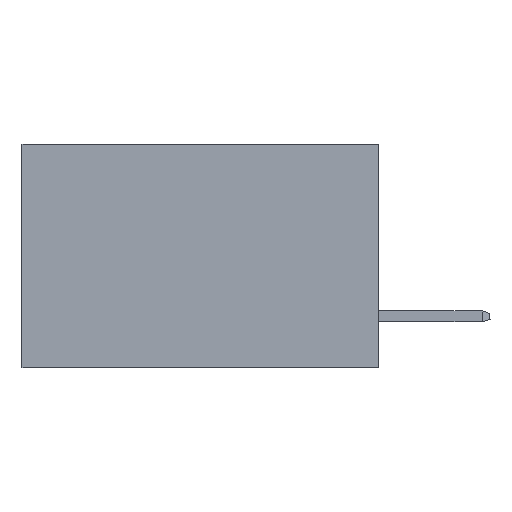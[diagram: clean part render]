
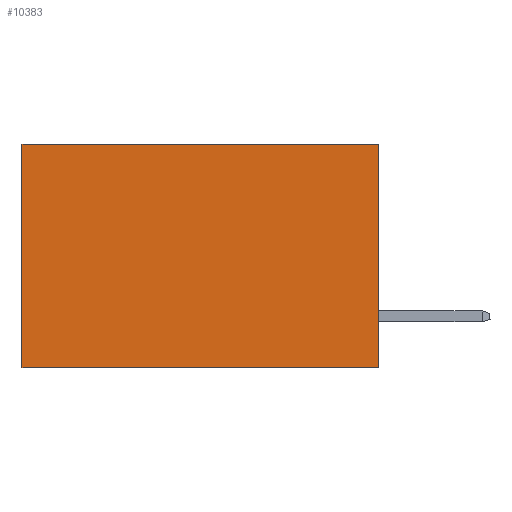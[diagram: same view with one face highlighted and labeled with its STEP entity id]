
A CAD part, left-side view. The second image highlights one B-rep face of the part: STEP entity #10383.
In plain terms, the highlighted planar face has unit normal (-1, 0, 0).
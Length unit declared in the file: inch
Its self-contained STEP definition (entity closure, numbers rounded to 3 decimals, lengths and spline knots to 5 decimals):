
#186 = LINE ( 'NONE', #8048, #23563 ) ;
#542 = DIRECTION ( 'NONE',  ( 0., 0., -1. ) ) ;
#1383 = DIRECTION ( 'NONE',  ( 1., 0., 0. ) ) ;
#2556 = AXIS2_PLACEMENT_3D ( 'NONE', #6354, #1383, #23823 ) ;
#4753 = CARTESIAN_POINT ( 'NONE',  ( 0.277, 0., 0. ) ) ;
#6354 = CARTESIAN_POINT ( 'NONE',  ( 0.277, 0., -0.37 ) ) ;
#8048 = CARTESIAN_POINT ( 'NONE',  ( 0.277, 0., -0.37 ) ) ;
#8263 = VERTEX_POINT ( 'NONE', #22224 ) ;
#8755 = PLANE ( 'NONE',  #2556 ) ;
#8800 = ORIENTED_EDGE ( 'NONE', *, *, #22665, .T. ) ;
#9054 = EDGE_CURVE ( 'NONE', #21464, #21645, #18186, .T. ) ;
#9182 = ORIENTED_EDGE ( 'NONE', *, *, #14695, .F. ) ;
#9859 = ORIENTED_EDGE ( 'NONE', *, *, #22012, .F. ) ;
#10264 = VERTEX_POINT ( 'NONE', #21380 ) ;
#10383 = ADVANCED_FACE ( 'NONE', ( #13274 ), #8755, .F. ) ;
#10411 = CARTESIAN_POINT ( 'NONE',  ( 0.277, 0.59, 0. ) ) ;
#13274 = FACE_OUTER_BOUND ( 'NONE', #14741, .T. ) ;
#13342 = VECTOR ( 'NONE', #13532, 39.37008 ) ;
#13532 = DIRECTION ( 'NONE',  ( 0., 0., -1. ) ) ;
#13721 = VECTOR ( 'NONE', #15578, 39.37008 ) ;
#13754 = CARTESIAN_POINT ( 'NONE',  ( 0.277, 0., -0.37 ) ) ;
#13959 = CARTESIAN_POINT ( 'NONE',  ( 0.277, 0.59, -0.37 ) ) ;
#14559 = VECTOR ( 'NONE', #19463, 39.37008 ) ;
#14695 = EDGE_CURVE ( 'NONE', #8263, #10264, #186, .T. ) ;
#14741 = EDGE_LOOP ( 'NONE', ( #23650, #9859, #9182, #8800 ) ) ;
#15114 = LINE ( 'NONE', #4753, #14559 ) ;
#15578 = DIRECTION ( 'NONE',  ( 0., 1., 0. ) ) ;
#16402 = CARTESIAN_POINT ( 'NONE',  ( 0.277, 0.59, -0.37 ) ) ;
#18186 = LINE ( 'NONE', #13959, #13342 ) ;
#19463 = DIRECTION ( 'NONE',  ( 0., 1., 0. ) ) ;
#21380 = CARTESIAN_POINT ( 'NONE',  ( 0.277, 0., -0.37 ) ) ;
#21464 = VERTEX_POINT ( 'NONE', #10411 ) ;
#21645 = VERTEX_POINT ( 'NONE', #16402 ) ;
#22012 = EDGE_CURVE ( 'NONE', #10264, #21645, #23341, .T. ) ;
#22224 = CARTESIAN_POINT ( 'NONE',  ( 0.277, 0., 0. ) ) ;
#22665 = EDGE_CURVE ( 'NONE', #8263, #21464, #15114, .T. ) ;
#23341 = LINE ( 'NONE', #13754, #13721 ) ;
#23563 = VECTOR ( 'NONE', #542, 39.37008 ) ;
#23650 = ORIENTED_EDGE ( 'NONE', *, *, #9054, .T. ) ;
#23823 = DIRECTION ( 'NONE',  ( 0., 0., -1. ) ) ;
